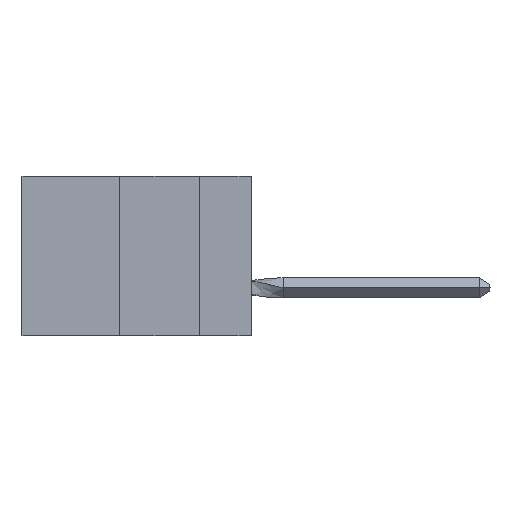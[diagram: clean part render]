
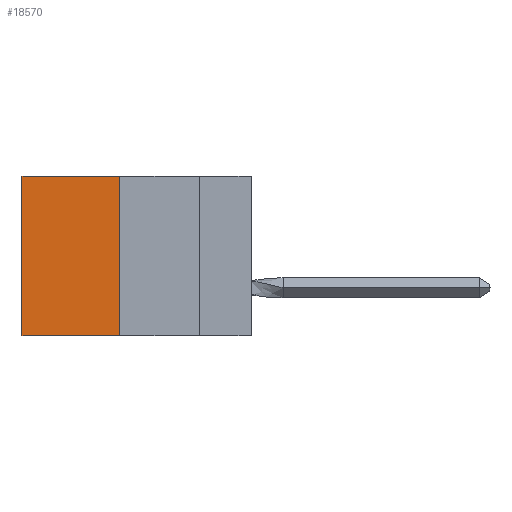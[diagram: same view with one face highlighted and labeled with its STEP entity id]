
A CAD part, left-side view. The second image highlights one B-rep face of the part: STEP entity #18570.
In plain terms, the highlighted planar face has unit normal (-1, 0, 0).
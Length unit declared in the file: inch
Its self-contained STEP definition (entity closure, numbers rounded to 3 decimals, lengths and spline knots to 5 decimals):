
#299 = ORIENTED_EDGE ( 'NONE', *, *, #4973, .F. ) ;
#2513 = DIRECTION ( 'NONE',  ( 0., 0., -1. ) ) ;
#3052 = DIRECTION ( 'NONE',  ( 0., 0., -1. ) ) ;
#3261 = CARTESIAN_POINT ( 'NONE',  ( 0.305, 0.413, -0.5 ) ) ;
#3486 = EDGE_CURVE ( 'NONE', #11361, #13059, #20712, .T. ) ;
#3859 = VECTOR ( 'NONE', #8205, 39.37008 ) ;
#4973 = EDGE_CURVE ( 'NONE', #11361, #8104, #5313, .T. ) ;
#4986 = EDGE_LOOP ( 'NONE', ( #17065, #18072, #299, #19717 ) ) ;
#5150 = EDGE_CURVE ( 'NONE', #13059, #17258, #14848, .T. ) ;
#5313 = LINE ( 'NONE', #22407, #12843 ) ;
#6705 = CARTESIAN_POINT ( 'NONE',  ( 0.305, 0.413, -0.5 ) ) ;
#7501 = CARTESIAN_POINT ( 'NONE',  ( 0.305, 0.413, 0. ) ) ;
#8013 = CARTESIAN_POINT ( 'NONE',  ( 0.305, 0.413, 0. ) ) ;
#8104 = VERTEX_POINT ( 'NONE', #3261 ) ;
#8205 = DIRECTION ( 'NONE',  ( 0., 0., -1. ) ) ;
#8844 = VECTOR ( 'NONE', #9373, 39.37008 ) ;
#9016 = FACE_OUTER_BOUND ( 'NONE', #4986, .T. ) ;
#9373 = DIRECTION ( 'NONE',  ( 0., 1., 0. ) ) ;
#9937 = AXIS2_PLACEMENT_3D ( 'NONE', #6705, #21496, #3052 ) ;
#10025 = CARTESIAN_POINT ( 'NONE',  ( 0.305, 0.413, -0.5 ) ) ;
#11160 = CARTESIAN_POINT ( 'NONE',  ( 0.305, 0.72, 0. ) ) ;
#11192 = LINE ( 'NONE', #10025, #21606 ) ;
#11361 = VERTEX_POINT ( 'NONE', #8013 ) ;
#12843 = VECTOR ( 'NONE', #2513, 39.37008 ) ;
#13059 = VERTEX_POINT ( 'NONE', #11160 ) ;
#13350 = EDGE_CURVE ( 'NONE', #8104, #17258, #11192, .T. ) ;
#13719 = CARTESIAN_POINT ( 'NONE',  ( 0.305, 0.72, -0.5 ) ) ;
#14848 = LINE ( 'NONE', #13719, #3859 ) ;
#15666 = CARTESIAN_POINT ( 'NONE',  ( 0.305, 0.72, -0.5 ) ) ;
#15720 = DIRECTION ( 'NONE',  ( 0., 1., 0. ) ) ;
#17065 = ORIENTED_EDGE ( 'NONE', *, *, #5150, .T. ) ;
#17258 = VERTEX_POINT ( 'NONE', #15666 ) ;
#17794 = PLANE ( 'NONE',  #9937 ) ;
#18072 = ORIENTED_EDGE ( 'NONE', *, *, #13350, .F. ) ;
#18570 = ADVANCED_FACE ( 'NONE', ( #9016 ), #17794, .F. ) ;
#19717 = ORIENTED_EDGE ( 'NONE', *, *, #3486, .T. ) ;
#20712 = LINE ( 'NONE', #7501, #8844 ) ;
#21496 = DIRECTION ( 'NONE',  ( 1., 0., 0. ) ) ;
#21606 = VECTOR ( 'NONE', #15720, 39.37008 ) ;
#22407 = CARTESIAN_POINT ( 'NONE',  ( 0.305, 0.413, -0.5 ) ) ;
